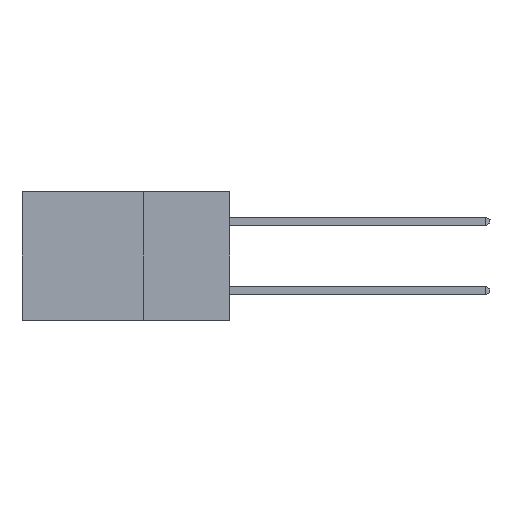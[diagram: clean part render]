
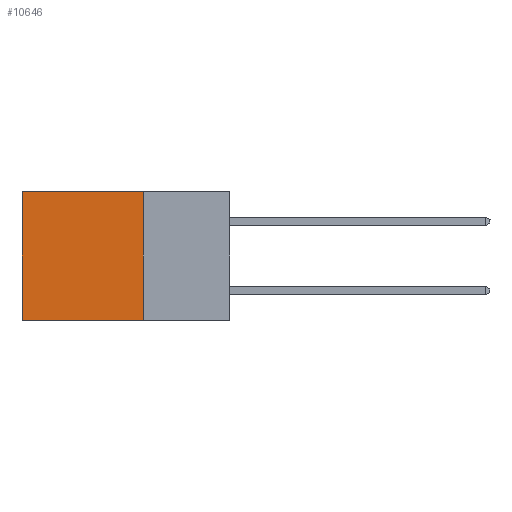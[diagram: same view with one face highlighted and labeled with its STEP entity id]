
A CAD part, left-side view. The second image highlights one B-rep face of the part: STEP entity #10646.
In plain terms, the highlighted planar face has unit normal (-1, 0, 0).
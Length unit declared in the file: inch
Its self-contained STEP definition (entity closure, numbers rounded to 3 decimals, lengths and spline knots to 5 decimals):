
#129 = ORIENTED_EDGE ( 'NONE', *, *, #15750, .T. ) ;
#265 = CARTESIAN_POINT ( 'NONE',  ( 0.298, 0.6, -0.37 ) ) ;
#672 = DIRECTION ( 'NONE',  ( 0., 1., 0. ) ) ;
#933 = EDGE_CURVE ( 'NONE', #4860, #10652, #14039, .T. ) ;
#1235 = EDGE_CURVE ( 'NONE', #19760, #15913, #16274, .T. ) ;
#1560 = VECTOR ( 'NONE', #5833, 39.37008 ) ;
#1700 = ORIENTED_EDGE ( 'NONE', *, *, #1235, .T. ) ;
#1740 = EDGE_LOOP ( 'NONE', ( #129, #7702, #10212, #1700 ) ) ;
#1744 = PLANE ( 'NONE',  #7239 ) ;
#2577 = FACE_OUTER_BOUND ( 'NONE', #1740, .T. ) ;
#4210 = CARTESIAN_POINT ( 'NONE',  ( 0.298, 0.6, 0. ) ) ;
#4860 = VERTEX_POINT ( 'NONE', #8236 ) ;
#5114 = DIRECTION ( 'NONE',  ( 1., 0., 0. ) ) ;
#5833 = DIRECTION ( 'NONE',  ( 0., 0., -1. ) ) ;
#7239 = AXIS2_PLACEMENT_3D ( 'NONE', #14682, #5114, #16324 ) ;
#7310 = EDGE_CURVE ( 'NONE', #19760, #4860, #12825, .T. ) ;
#7686 = DIRECTION ( 'NONE',  ( 0., 0., -1. ) ) ;
#7702 = ORIENTED_EDGE ( 'NONE', *, *, #933, .F. ) ;
#8236 = CARTESIAN_POINT ( 'NONE',  ( 0.298, 0.25, -0.37 ) ) ;
#8748 = VECTOR ( 'NONE', #672, 39.37008 ) ;
#9031 = CARTESIAN_POINT ( 'NONE',  ( 0.298, 0.25, 0. ) ) ;
#10212 = ORIENTED_EDGE ( 'NONE', *, *, #7310, .F. ) ;
#10453 = CARTESIAN_POINT ( 'NONE',  ( 0.298, 0.25, -0.37 ) ) ;
#10646 = ADVANCED_FACE ( 'NONE', ( #2577 ), #1744, .F. ) ;
#10652 = VERTEX_POINT ( 'NONE', #265 ) ;
#12825 = LINE ( 'NONE', #9031, #15336 ) ;
#13350 = CARTESIAN_POINT ( 'NONE',  ( 0.298, 0.25, 0. ) ) ;
#13620 = DIRECTION ( 'NONE',  ( 0., 1., 0. ) ) ;
#14039 = LINE ( 'NONE', #10453, #8748 ) ;
#14682 = CARTESIAN_POINT ( 'NONE',  ( 0.298, 0.25, 0. ) ) ;
#15336 = VECTOR ( 'NONE', #7686, 39.37008 ) ;
#15750 = EDGE_CURVE ( 'NONE', #15913, #10652, #19718, .T. ) ;
#15913 = VERTEX_POINT ( 'NONE', #18581 ) ;
#16274 = LINE ( 'NONE', #13350, #17072 ) ;
#16324 = DIRECTION ( 'NONE',  ( 0., 0., -1. ) ) ;
#17072 = VECTOR ( 'NONE', #13620, 39.37008 ) ;
#18581 = CARTESIAN_POINT ( 'NONE',  ( 0.298, 0.6, 0. ) ) ;
#19644 = CARTESIAN_POINT ( 'NONE',  ( 0.298, 0.25, 0. ) ) ;
#19718 = LINE ( 'NONE', #4210, #1560 ) ;
#19760 = VERTEX_POINT ( 'NONE', #19644 ) ;
